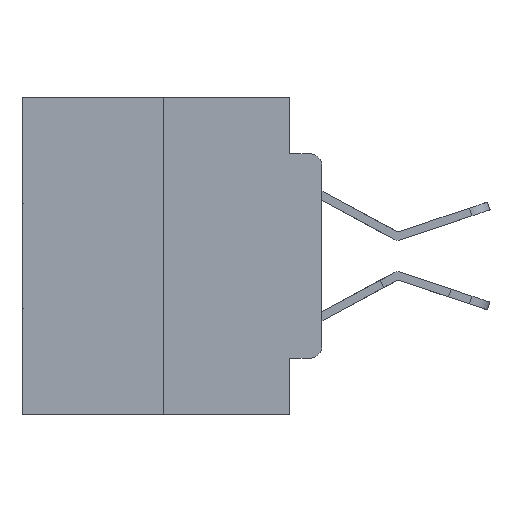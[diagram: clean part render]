
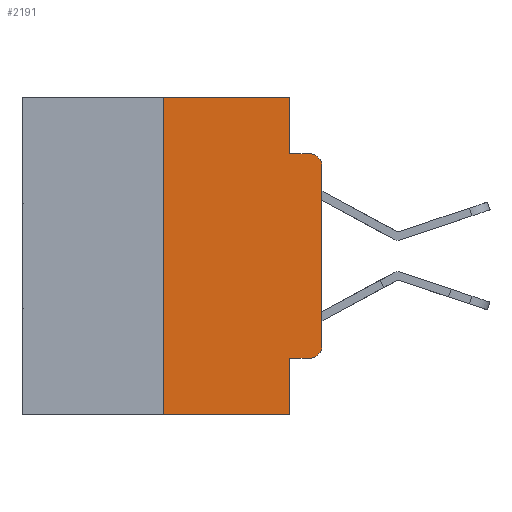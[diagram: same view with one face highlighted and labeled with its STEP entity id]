
A CAD part, left-side view. The second image highlights one B-rep face of the part: STEP entity #2191.
In plain terms, the highlighted planar face has unit normal (-1, 0, 0).
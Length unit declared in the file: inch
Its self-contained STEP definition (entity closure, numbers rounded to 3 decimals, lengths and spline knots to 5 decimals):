
#351 = DIRECTION ( 'NONE',  ( 1., 0., 0. ) ) ;
#699 = VERTEX_POINT ( 'NONE', #19082 ) ;
#701 = EDGE_CURVE ( 'NONE', #26719, #9493, #16705, .T. ) ;
#1190 = ORIENTED_EDGE ( 'NONE', *, *, #21058, .T. ) ;
#1380 = LINE ( 'NONE', #22360, #24370 ) ;
#1488 = DIRECTION ( 'NONE',  ( 0., 0., 1. ) ) ;
#1520 = DIRECTION ( 'NONE',  ( 0., 0., 1. ) ) ;
#2153 = DIRECTION ( 'NONE',  ( 0., 0., -1. ) ) ;
#2191 = ADVANCED_FACE ( 'NONE', ( #25454 ), #13587, .F. ) ;
#2335 = AXIS2_PLACEMENT_3D ( 'NONE', #16698, #351, #2153 ) ;
#2825 = CARTESIAN_POINT ( 'NONE',  ( 0., 0.051, -0.5 ) ) ;
#2838 = EDGE_CURVE ( 'NONE', #26719, #24290, #5189, .T. ) ;
#2999 = DIRECTION ( 'NONE',  ( -1., 0., 0. ) ) ;
#3312 = CARTESIAN_POINT ( 'NONE',  ( 0., 0.473, 0. ) ) ;
#3818 = VERTEX_POINT ( 'NONE', #22117 ) ;
#4025 = DIRECTION ( 'NONE',  ( 0., -1., 0. ) ) ;
#5016 = LINE ( 'NONE', #18564, #22868 ) ;
#5189 = LINE ( 'NONE', #8168, #22022 ) ;
#5296 = VECTOR ( 'NONE', #1520, 39.37008 ) ;
#5649 = VECTOR ( 'NONE', #1488, 39.37008 ) ;
#5780 = ORIENTED_EDGE ( 'NONE', *, *, #21959, .F. ) ;
#6154 = EDGE_LOOP ( 'NONE', ( #21432, #6405, #28029, #6996, #25663, #10869, #23535, #5780, #21189, #1190 ) ) ;
#6187 = CARTESIAN_POINT ( 'NONE',  ( 0., 0.25, 0. ) ) ;
#6405 = ORIENTED_EDGE ( 'NONE', *, *, #11544, .T. ) ;
#6611 = DIRECTION ( 'NONE',  ( 0., 0., -1. ) ) ;
#6802 = DIRECTION ( 'NONE',  ( -1., 0., 0. ) ) ;
#6996 = ORIENTED_EDGE ( 'NONE', *, *, #27876, .F. ) ;
#7298 = CIRCLE ( 'NONE', #15806, 0.02 ) ;
#7332 = CARTESIAN_POINT ( 'NONE',  ( 0., 0.25, -0.5 ) ) ;
#7397 = VERTEX_POINT ( 'NONE', #7477 ) ;
#7477 = CARTESIAN_POINT ( 'NONE',  ( 0., 0.051, -0.0885 ) ) ;
#8168 = CARTESIAN_POINT ( 'NONE',  ( 0., 0.473, -0.5 ) ) ;
#8489 = CARTESIAN_POINT ( 'NONE',  ( 0., 0.25, 0. ) ) ;
#9224 = DIRECTION ( 'NONE',  ( 0., 0., -1. ) ) ;
#9341 = DIRECTION ( 'NONE',  ( 0., -1., 0. ) ) ;
#9493 = VERTEX_POINT ( 'NONE', #8489 ) ;
#9783 = DIRECTION ( 'NONE',  ( 0., -1., 0. ) ) ;
#10114 = VECTOR ( 'NONE', #9783, 39.37008 ) ;
#10869 = ORIENTED_EDGE ( 'NONE', *, *, #701, .F. ) ;
#11544 = EDGE_CURVE ( 'NONE', #13705, #19560, #7298, .T. ) ;
#12144 = VECTOR ( 'NONE', #14558, 39.37008 ) ;
#12544 = LINE ( 'NONE', #19857, #5296 ) ;
#13587 = PLANE ( 'NONE',  #2335 ) ;
#13705 = VERTEX_POINT ( 'NONE', #17394 ) ;
#14006 = CARTESIAN_POINT ( 'NONE',  ( 0., 0.02, -0.0885 ) ) ;
#14457 = LINE ( 'NONE', #23297, #16933 ) ;
#14558 = DIRECTION ( 'NONE',  ( 0., -1., 0. ) ) ;
#15806 = AXIS2_PLACEMENT_3D ( 'NONE', #16195, #2999, #18395 ) ;
#15949 = LINE ( 'NONE', #18325, #10114 ) ;
#16195 = CARTESIAN_POINT ( 'NONE',  ( 0., 0.02, -0.1085 ) ) ;
#16698 = CARTESIAN_POINT ( 'NONE',  ( 0., 0.473, 0. ) ) ;
#16705 = LINE ( 'NONE', #6187, #5649 ) ;
#16933 = VECTOR ( 'NONE', #22926, 39.37008 ) ;
#17187 = VERTEX_POINT ( 'NONE', #20392 ) ;
#17394 = CARTESIAN_POINT ( 'NONE',  ( 0., 0., -0.1085 ) ) ;
#17887 = EDGE_CURVE ( 'NONE', #699, #17187, #5016, .T. ) ;
#18325 = CARTESIAN_POINT ( 'NONE',  ( 0., 0.051, -0.0885 ) ) ;
#18395 = DIRECTION ( 'NONE',  ( 0., 0., -1. ) ) ;
#18564 = CARTESIAN_POINT ( 'NONE',  ( 0., 0.051, -0.4115 ) ) ;
#18966 = VERTEX_POINT ( 'NONE', #20657 ) ;
#19023 = CIRCLE ( 'NONE', #21123, 0.02 ) ;
#19082 = CARTESIAN_POINT ( 'NONE',  ( 0., 0.051, -0.4115 ) ) ;
#19560 = VERTEX_POINT ( 'NONE', #14006 ) ;
#19848 = CARTESIAN_POINT ( 'NONE',  ( 0., 0.02, -0.3915 ) ) ;
#19857 = CARTESIAN_POINT ( 'NONE',  ( 0., 0., 0. ) ) ;
#19901 = EDGE_CURVE ( 'NONE', #3818, #13705, #12544, .T. ) ;
#20392 = CARTESIAN_POINT ( 'NONE',  ( 0., 0.02, -0.4115 ) ) ;
#20657 = CARTESIAN_POINT ( 'NONE',  ( 0., 0.051, 0. ) ) ;
#21058 = EDGE_CURVE ( 'NONE', #17187, #3818, #19023, .T. ) ;
#21123 = AXIS2_PLACEMENT_3D ( 'NONE', #19848, #6802, #6611 ) ;
#21189 = ORIENTED_EDGE ( 'NONE', *, *, #17887, .T. ) ;
#21432 = ORIENTED_EDGE ( 'NONE', *, *, #19901, .T. ) ;
#21959 = EDGE_CURVE ( 'NONE', #699, #24290, #14457, .T. ) ;
#22022 = VECTOR ( 'NONE', #4025, 39.37008 ) ;
#22117 = CARTESIAN_POINT ( 'NONE',  ( 0., 0., -0.3915 ) ) ;
#22360 = CARTESIAN_POINT ( 'NONE',  ( 0., 0.051, 0. ) ) ;
#22868 = VECTOR ( 'NONE', #9341, 39.37008 ) ;
#22926 = DIRECTION ( 'NONE',  ( 0., 0., -1. ) ) ;
#23297 = CARTESIAN_POINT ( 'NONE',  ( 0., 0.051, 0. ) ) ;
#23535 = ORIENTED_EDGE ( 'NONE', *, *, #2838, .T. ) ;
#24290 = VERTEX_POINT ( 'NONE', #2825 ) ;
#24370 = VECTOR ( 'NONE', #9224, 39.37008 ) ;
#25454 = FACE_OUTER_BOUND ( 'NONE', #6154, .T. ) ;
#25663 = ORIENTED_EDGE ( 'NONE', *, *, #26316, .F. ) ;
#26186 = EDGE_CURVE ( 'NONE', #7397, #19560, #15949, .T. ) ;
#26316 = EDGE_CURVE ( 'NONE', #9493, #18966, #27537, .T. ) ;
#26719 = VERTEX_POINT ( 'NONE', #7332 ) ;
#27537 = LINE ( 'NONE', #3312, #12144 ) ;
#27876 = EDGE_CURVE ( 'NONE', #18966, #7397, #1380, .T. ) ;
#28029 = ORIENTED_EDGE ( 'NONE', *, *, #26186, .F. ) ;
